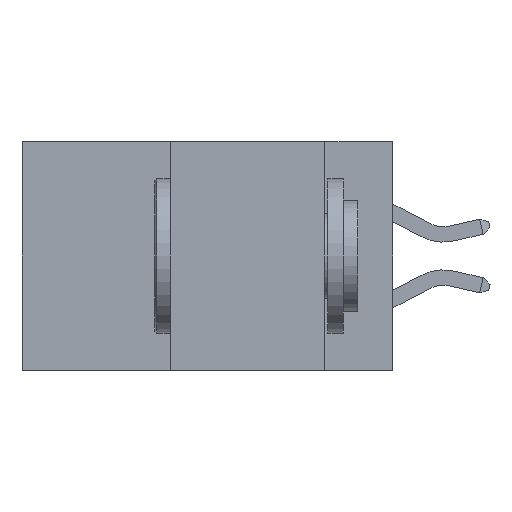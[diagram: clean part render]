
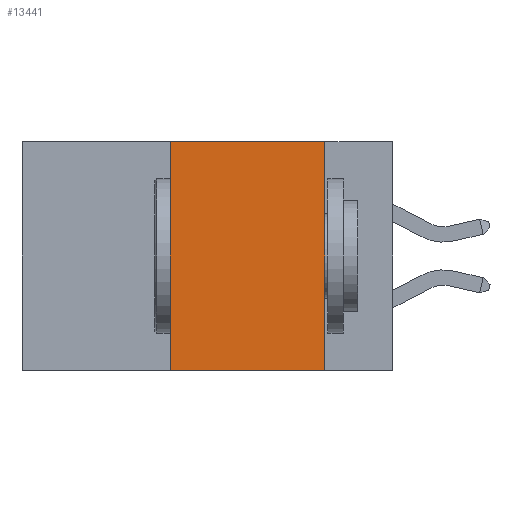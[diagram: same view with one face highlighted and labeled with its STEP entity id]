
A CAD part, left-side view. The second image highlights one B-rep face of the part: STEP entity #13441.
In plain terms, the highlighted planar face has unit normal (-1, 0, 0).
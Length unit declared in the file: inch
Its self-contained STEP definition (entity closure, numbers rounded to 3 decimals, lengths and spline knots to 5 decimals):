
#128 = EDGE_CURVE ( 'NONE', #529, #8367, #3109, .T. ) ;
#183 = LINE ( 'NONE', #19446, #19087 ) ;
#529 = VERTEX_POINT ( 'NONE', #22422 ) ;
#1268 = EDGE_CURVE ( 'NONE', #11169, #7626, #13112, .T. ) ;
#1272 = DIRECTION ( 'NONE',  ( 0., -1., 0. ) ) ;
#2907 = CARTESIAN_POINT ( 'NONE',  ( 0., 0.6, -0.37 ) ) ;
#3109 = LINE ( 'NONE', #17085, #12920 ) ;
#3822 = EDGE_CURVE ( 'NONE', #11169, #529, #183, .T. ) ;
#4239 = ORIENTED_EDGE ( 'NONE', *, *, #10003, .F. ) ;
#5145 = CARTESIAN_POINT ( 'NONE',  ( 0., 0.11, 0. ) ) ;
#6782 = ORIENTED_EDGE ( 'NONE', *, *, #128, .F. ) ;
#7626 = VERTEX_POINT ( 'NONE', #8337 ) ;
#7851 = FACE_OUTER_BOUND ( 'NONE', #20484, .T. ) ;
#8337 = CARTESIAN_POINT ( 'NONE',  ( 0., 0.11, -0.37 ) ) ;
#8367 = VERTEX_POINT ( 'NONE', #23176 ) ;
#8458 = PLANE ( 'NONE',  #17733 ) ;
#10003 = EDGE_CURVE ( 'NONE', #8367, #7626, #10506, .T. ) ;
#10225 = ORIENTED_EDGE ( 'NONE', *, *, #1268, .T. ) ;
#10281 = DIRECTION ( 'NONE',  ( 1., 0., 0. ) ) ;
#10506 = LINE ( 'NONE', #5145, #14729 ) ;
#11169 = VERTEX_POINT ( 'NONE', #21287 ) ;
#12121 = DIRECTION ( 'NONE',  ( 0., -1., 0. ) ) ;
#12246 = ORIENTED_EDGE ( 'NONE', *, *, #3822, .F. ) ;
#12920 = VECTOR ( 'NONE', #12121, 39.37008 ) ;
#13112 = LINE ( 'NONE', #2907, #13682 ) ;
#13441 = ADVANCED_FACE ( 'NONE', ( #7851 ), #8458, .F. ) ;
#13682 = VECTOR ( 'NONE', #1272, 39.37008 ) ;
#14729 = VECTOR ( 'NONE', #16088, 39.37008 ) ;
#15969 = DIRECTION ( 'NONE',  ( 0., 0., 1. ) ) ;
#16088 = DIRECTION ( 'NONE',  ( 0., 0., -1. ) ) ;
#17085 = CARTESIAN_POINT ( 'NONE',  ( 0., 0.6, 0. ) ) ;
#17733 = AXIS2_PLACEMENT_3D ( 'NONE', #20915, #10281, #22659 ) ;
#19087 = VECTOR ( 'NONE', #15969, 39.37008 ) ;
#19446 = CARTESIAN_POINT ( 'NONE',  ( 0., 0.36, 0. ) ) ;
#20484 = EDGE_LOOP ( 'NONE', ( #4239, #6782, #12246, #10225 ) ) ;
#20915 = CARTESIAN_POINT ( 'NONE',  ( 0., 0.6, 0. ) ) ;
#21287 = CARTESIAN_POINT ( 'NONE',  ( 0., 0.36, -0.37 ) ) ;
#22422 = CARTESIAN_POINT ( 'NONE',  ( 0., 0.36, 0. ) ) ;
#22659 = DIRECTION ( 'NONE',  ( 0., 0., -1. ) ) ;
#23176 = CARTESIAN_POINT ( 'NONE',  ( 0., 0.11, 0. ) ) ;
